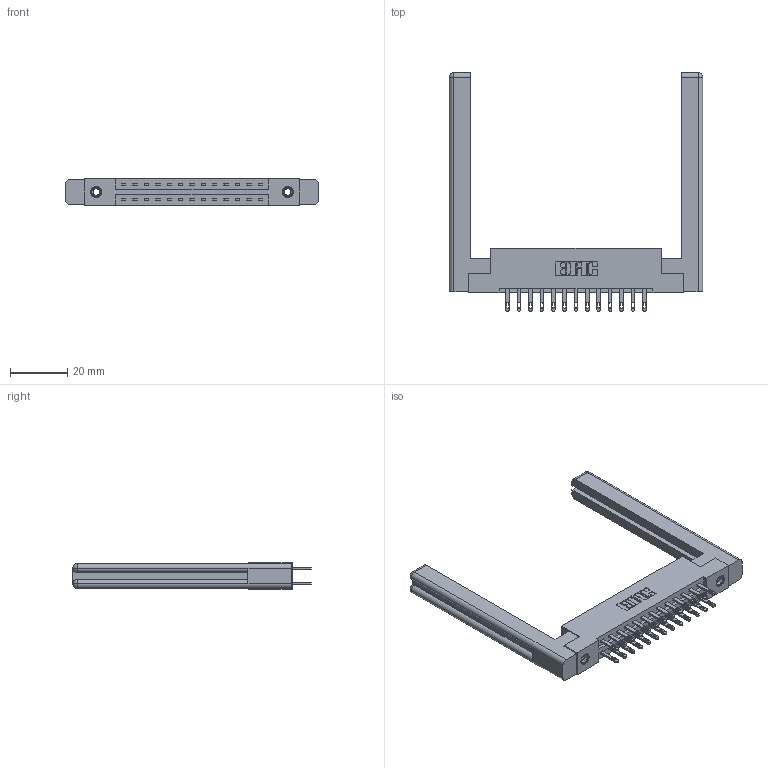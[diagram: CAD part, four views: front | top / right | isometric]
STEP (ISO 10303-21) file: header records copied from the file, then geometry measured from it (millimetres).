
FILE_DESCRIPTION (( 'STEP AP203' ), '1' );
FILE_NAME ('337-026-500-258.STEP', '2019-10-08T15:54:24', ( '' ), ( '' ), 'SwSTEP 2.0', 'SolidWorks 2016', '' );
FILE_SCHEMA (( 'CONFIG_CONTROL_DESIGN' ));
Length unit declared in the file: inch
Products named in the file (5): 337-026-500-258; 337 Part_Flush Mounting Lugs - 0.156 Dia-TI; 345-292-001_345-293-100; 307-220-058; 345-250-001_345-250-001-102
Assembly tree (31 placements, depth 2):
  337-026-500-258
    337 Part_Flush Mounting Lugs - 0.156 Dia-TI
    345-292-001_345-293-100  x26
    345-250-001_345-250-001-102  x2
    307-220-058  x2
Bounding box: 88.14 x 82.94 x 9.4 mm (x, y, z)
Volume: 16124.5 mm3; surface area: 15207.8 mm2
Topology: 31 solids, 31 shells, 1556 faces, 4643 edges, 3082 vertices
Faces by surface type: plane 986, cylinder 546, cone 12, torus 12
Entity records: 16394 total; most frequent: CARTESIAN_POINT 2793, ORIENTED_EDGE 2668, DIRECTION 2446, EDGE_CURVE 1334, LINE 1154, VECTOR 1154, VERTEX_POINT 882, AXIS2_PLACEMENT_3D 646
